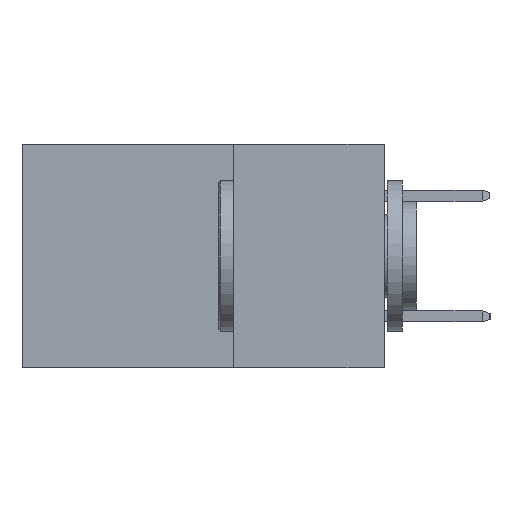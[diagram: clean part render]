
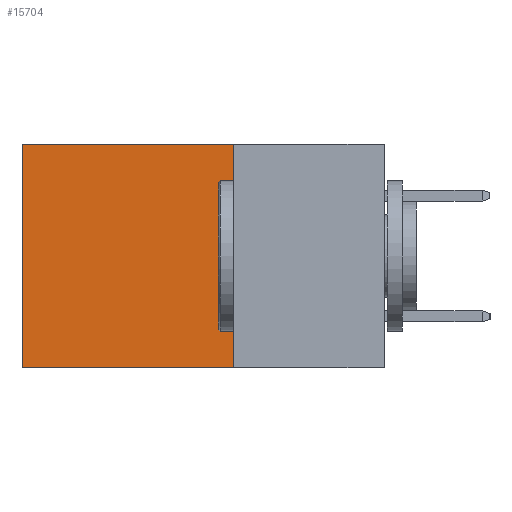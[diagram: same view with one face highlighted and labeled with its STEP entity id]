
A CAD part, left-side view. The second image highlights one B-rep face of the part: STEP entity #15704.
In plain terms, the highlighted planar face has unit normal (-1, 0, 0).
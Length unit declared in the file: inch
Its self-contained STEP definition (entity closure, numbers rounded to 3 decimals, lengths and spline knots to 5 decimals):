
#599 = VERTEX_POINT ( 'NONE', #11448 ) ;
#1033 = LINE ( 'NONE', #15684, #14990 ) ;
#2265 = DIRECTION ( 'NONE',  ( 0., 0., -1. ) ) ;
#2303 = CARTESIAN_POINT ( 'NONE',  ( 0.2615, 0.25, -0.37 ) ) ;
#2615 = AXIS2_PLACEMENT_3D ( 'NONE', #16640, #10219, #2265 ) ;
#2652 = VECTOR ( 'NONE', #11608, 39.37008 ) ;
#3336 = VERTEX_POINT ( 'NONE', #11799 ) ;
#4004 = DIRECTION ( 'NONE',  ( 0., 0., -1. ) ) ;
#4097 = VERTEX_POINT ( 'NONE', #6069 ) ;
#5268 = CARTESIAN_POINT ( 'NONE',  ( 0.2615, 0.25, -0.37 ) ) ;
#5869 = ORIENTED_EDGE ( 'NONE', *, *, #9734, .F. ) ;
#6069 = CARTESIAN_POINT ( 'NONE',  ( 0.2615, 0.6, -0.37 ) ) ;
#6357 = LINE ( 'NONE', #11942, #9888 ) ;
#6559 = ORIENTED_EDGE ( 'NONE', *, *, #16565, .T. ) ;
#6592 = DIRECTION ( 'NONE',  ( 0., 0., -1. ) ) ;
#7260 = EDGE_LOOP ( 'NONE', ( #6559, #5869, #16552, #10967 ) ) ;
#7918 = DIRECTION ( 'NONE',  ( 0., 1., 0. ) ) ;
#8409 = EDGE_CURVE ( 'NONE', #599, #9073, #1033, .T. ) ;
#9073 = VERTEX_POINT ( 'NONE', #10266 ) ;
#9734 = EDGE_CURVE ( 'NONE', #3336, #4097, #13204, .T. ) ;
#9888 = VECTOR ( 'NONE', #4004, 39.37008 ) ;
#9913 = EDGE_CURVE ( 'NONE', #599, #3336, #10779, .T. ) ;
#10219 = DIRECTION ( 'NONE',  ( 1., 0., 0. ) ) ;
#10266 = CARTESIAN_POINT ( 'NONE',  ( 0.2615, 0.6, 0. ) ) ;
#10779 = LINE ( 'NONE', #5268, #13772 ) ;
#10967 = ORIENTED_EDGE ( 'NONE', *, *, #8409, .T. ) ;
#11448 = CARTESIAN_POINT ( 'NONE',  ( 0.2615, 0.25, 0. ) ) ;
#11608 = DIRECTION ( 'NONE',  ( 0., 1., 0. ) ) ;
#11799 = CARTESIAN_POINT ( 'NONE',  ( 0.2615, 0.25, -0.37 ) ) ;
#11942 = CARTESIAN_POINT ( 'NONE',  ( 0.2615, 0.6, -0.37 ) ) ;
#13204 = LINE ( 'NONE', #2303, #2652 ) ;
#13772 = VECTOR ( 'NONE', #6592, 39.37008 ) ;
#14990 = VECTOR ( 'NONE', #7918, 39.37008 ) ;
#15319 = PLANE ( 'NONE',  #2615 ) ;
#15684 = CARTESIAN_POINT ( 'NONE',  ( 0.2615, 0.25, 0. ) ) ;
#15704 = ADVANCED_FACE ( 'NONE', ( #16794 ), #15319, .F. ) ;
#16552 = ORIENTED_EDGE ( 'NONE', *, *, #9913, .F. ) ;
#16565 = EDGE_CURVE ( 'NONE', #9073, #4097, #6357, .T. ) ;
#16640 = CARTESIAN_POINT ( 'NONE',  ( 0.2615, 0.25, -0.37 ) ) ;
#16794 = FACE_OUTER_BOUND ( 'NONE', #7260, .T. ) ;
